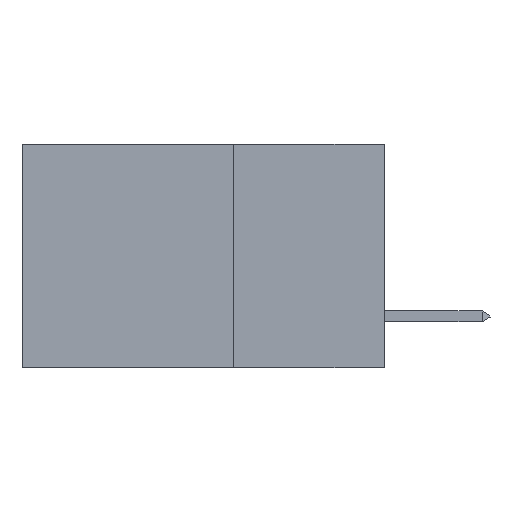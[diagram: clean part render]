
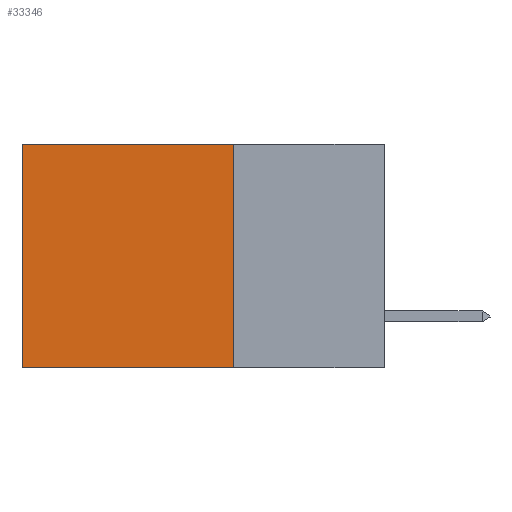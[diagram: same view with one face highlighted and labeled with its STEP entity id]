
A CAD part, left-side view. The second image highlights one B-rep face of the part: STEP entity #33346.
In plain terms, the highlighted planar face has unit normal (-1, 0, 0).
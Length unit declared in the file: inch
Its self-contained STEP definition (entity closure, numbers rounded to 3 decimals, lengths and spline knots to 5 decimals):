
#2225 = VECTOR ( 'NONE', #15639, 39.37008 ) ;
#2235 = CARTESIAN_POINT ( 'NONE',  ( 0.2875, 0.25, 0. ) ) ;
#3206 = EDGE_CURVE ( 'NONE', #17196, #14304, #13713, .T. ) ;
#4710 = DIRECTION ( 'NONE',  ( 0., 1., 0. ) ) ;
#5265 = ORIENTED_EDGE ( 'NONE', *, *, #38005, .F. ) ;
#5830 = LINE ( 'NONE', #22402, #27474 ) ;
#9877 = EDGE_CURVE ( 'NONE', #34212, #17196, #38574, .T. ) ;
#11485 = CARTESIAN_POINT ( 'NONE',  ( 0.2875, 0.25, 0. ) ) ;
#12850 = CARTESIAN_POINT ( 'NONE',  ( 0.2875, 0.25, 0. ) ) ;
#13713 = LINE ( 'NONE', #34603, #2225 ) ;
#14304 = VERTEX_POINT ( 'NONE', #23121 ) ;
#14826 = AXIS2_PLACEMENT_3D ( 'NONE', #2235, #26962, #30043 ) ;
#15639 = DIRECTION ( 'NONE',  ( 0., 0., -1. ) ) ;
#16819 = CARTESIAN_POINT ( 'NONE',  ( 0.2875, 0.6, 0. ) ) ;
#17196 = VERTEX_POINT ( 'NONE', #16819 ) ;
#20157 = CARTESIAN_POINT ( 'NONE',  ( 0.2875, 0.25, -0.37 ) ) ;
#22402 = CARTESIAN_POINT ( 'NONE',  ( 0.2875, 0.25, 0. ) ) ;
#22728 = ORIENTED_EDGE ( 'NONE', *, *, #28989, .F. ) ;
#23121 = CARTESIAN_POINT ( 'NONE',  ( 0.2875, 0.6, -0.37 ) ) ;
#23712 = EDGE_LOOP ( 'NONE', ( #27082, #22728, #5265, #30450 ) ) ;
#24014 = PLANE ( 'NONE',  #14826 ) ;
#26962 = DIRECTION ( 'NONE',  ( 1., 0., 0. ) ) ;
#27082 = ORIENTED_EDGE ( 'NONE', *, *, #3206, .T. ) ;
#27474 = VECTOR ( 'NONE', #38068, 39.37008 ) ;
#28079 = DIRECTION ( 'NONE',  ( 0., 1., 0. ) ) ;
#28965 = VECTOR ( 'NONE', #28079, 39.37008 ) ;
#28989 = EDGE_CURVE ( 'NONE', #34291, #14304, #32901, .T. ) ;
#30043 = DIRECTION ( 'NONE',  ( 0., 0., -1. ) ) ;
#30450 = ORIENTED_EDGE ( 'NONE', *, *, #9877, .T. ) ;
#30845 = FACE_OUTER_BOUND ( 'NONE', #23712, .T. ) ;
#32736 = CARTESIAN_POINT ( 'NONE',  ( 0.2875, 0.25, -0.37 ) ) ;
#32901 = LINE ( 'NONE', #20157, #39639 ) ;
#33346 = ADVANCED_FACE ( 'NONE', ( #30845 ), #24014, .F. ) ;
#34212 = VERTEX_POINT ( 'NONE', #11485 ) ;
#34291 = VERTEX_POINT ( 'NONE', #32736 ) ;
#34603 = CARTESIAN_POINT ( 'NONE',  ( 0.2875, 0.6, 0. ) ) ;
#38005 = EDGE_CURVE ( 'NONE', #34212, #34291, #5830, .T. ) ;
#38068 = DIRECTION ( 'NONE',  ( 0., 0., -1. ) ) ;
#38574 = LINE ( 'NONE', #12850, #28965 ) ;
#39639 = VECTOR ( 'NONE', #4710, 39.37008 ) ;
